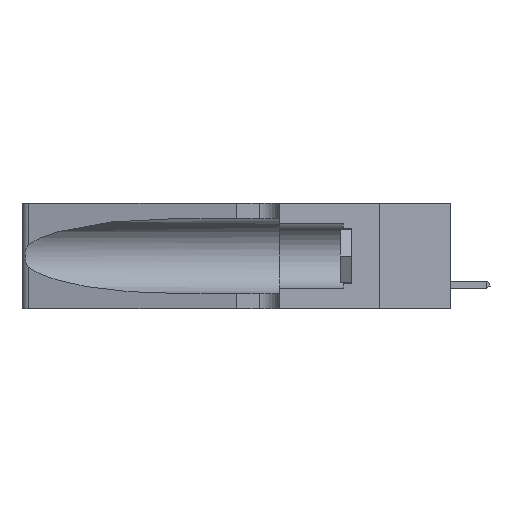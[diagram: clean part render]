
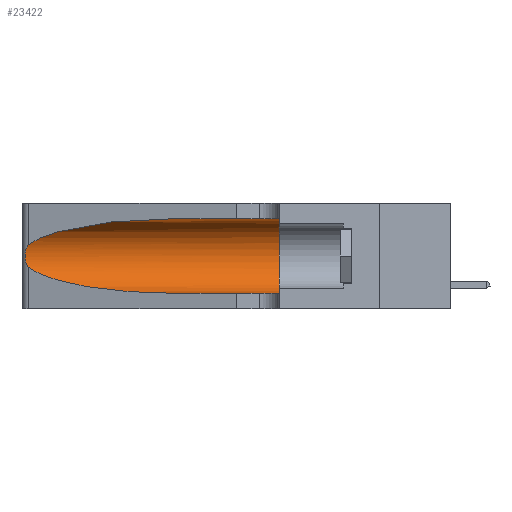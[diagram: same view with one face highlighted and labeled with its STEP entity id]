
A CAD part, left-side view. The second image highlights one B-rep face of the part: STEP entity #23422.
In plain terms, the highlighted cylindrical face has radius 3.308 mm (diameter 6.617 mm), a partial arc.
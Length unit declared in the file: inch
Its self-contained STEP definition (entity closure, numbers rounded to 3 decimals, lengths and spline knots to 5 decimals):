
#746 = ORIENTED_EDGE ( 'NONE', *, *, #5344, .F. ) ;
#1196 = CARTESIAN_POINT ( 'NONE',  ( 0.1305, 1.61858, 0.31525 ) ) ;
#1233 = VECTOR ( 'NONE', #22674, 39.37008 ) ;
#1549 = CARTESIAN_POINT ( 'NONE',  ( 0.25787, 1.23484, 0.2124 ) ) ;
#1666 = CARTESIAN_POINT ( 'NONE',  ( 0.25639, 1.23184, 0.21858 ) ) ;
#1991 = CARTESIAN_POINT ( 'NONE',  ( 0.1305, 0.72297, 0.05475 ) ) ;
#2087 = ORIENTED_EDGE ( 'NONE', *, *, #8302, .F. ) ;
#3786 = CARTESIAN_POINT ( 'NONE',  ( 0.18966, 0.96281, 0.31525 ) ) ;
#3876 = VERTEX_POINT ( 'NONE', #1991 ) ;
#3996 = VECTOR ( 'NONE', #4857, 39.37008 ) ;
#4454 = DIRECTION ( 'NONE',  ( 0., -1., 0. ) ) ;
#4857 = DIRECTION ( 'NONE',  ( 0., -1., 0. ) ) ;
#5344 = EDGE_CURVE ( 'NONE', #15802, #11603, #7976, .T. ) ;
#5470 = ORIENTED_EDGE ( 'NONE', *, *, #15708, .T. ) ;
#5559 = CARTESIAN_POINT ( 'NONE',  ( 0.25487, 1.22718, 0.22369 ) ) ;
#5665 = CARTESIAN_POINT ( 'NONE',  ( 0.25555, 1.22994, 0.2215 ) ) ;
#5696 = FACE_OUTER_BOUND ( 'NONE', #6865, .T. ) ;
#6238 = CARTESIAN_POINT ( 'NONE',  ( 0.25487, 1.22718, 0.22369 ) ) ;
#6282 = CARTESIAN_POINT ( 'NONE',  ( 0.25639, 1.23186, 0.15144 ) ) ;
#6865 = EDGE_LOOP ( 'NONE', ( #13003, #8755, #25587, #5470, #746, #2087 ) ) ;
#7184 = VERTEX_POINT ( 'NONE', #26812 ) ;
#7434 = CARTESIAN_POINT ( 'NONE',  ( 0.1305, 0.72297, 0.05475 ) ) ;
#7505 = CARTESIAN_POINT ( 'NONE',  ( 0.1305, 0.35, 0.185 ) ) ;
#7605 = DIRECTION ( 'NONE',  ( 0., 0., 1. ) ) ;
#7976 = CIRCLE ( 'NONE', #21541, 0.13025 ) ;
#8302 = EDGE_CURVE ( 'NONE', #19024, #15802, #31483, .T. ) ;
#8755 = ORIENTED_EDGE ( 'NONE', *, *, #11202, .T. ) ;
#8813 = CARTESIAN_POINT ( 'NONE',  ( 0.25487, 1.22718, 0.14631 ) ) ;
#9220 = CARTESIAN_POINT ( 'NONE',  ( 0.2373, 1.15595, 0.28018 ) ) ;
#9423 = CARTESIAN_POINT ( 'NONE',  ( 0.1305, 1.61858, 0.185 ) ) ;
#9803 =( BOUNDED_CURVE ( )  B_SPLINE_CURVE ( 3, ( #24480, #3786, #9220, #6238 ),
 .UNSPECIFIED., .F., .F. ) 
 B_SPLINE_CURVE_WITH_KNOTS ( ( 4, 4 ),
 ( 1.5708, 2.84003 ),
 .UNSPECIFIED. ) 
 CURVE ( )  GEOMETRIC_REPRESENTATION_ITEM ( )  RATIONAL_B_SPLINE_CURVE ( ( 1., 0.87, 0.87, 1. ) ) 
 REPRESENTATION_ITEM ( '' )  );
#11202 = EDGE_CURVE ( 'NONE', #28023, #7184, #19476, .T. ) ;
#11603 = VERTEX_POINT ( 'NONE', #31633 ) ;
#11711 = CARTESIAN_POINT ( 'NONE',  ( 0.26075, 1.23896, 0.19203 ) ) ;
#12378 = CARTESIAN_POINT ( 'NONE',  ( 0.1305, 1.61858, 0.05475 ) ) ;
#12766 = CARTESIAN_POINT ( 'NONE',  ( 0.25487, 1.22718, 0.22369 ) ) ;
#13003 = ORIENTED_EDGE ( 'NONE', *, *, #30274, .T. ) ;
#13230 = CYLINDRICAL_SURFACE ( 'NONE', #30563, 0.13025 ) ;
#15162 = CARTESIAN_POINT ( 'NONE',  ( 0.1305, 0.35, 0.31525 ) ) ;
#15708 = EDGE_CURVE ( 'NONE', #3876, #11603, #16445, .T. ) ;
#15802 = VERTEX_POINT ( 'NONE', #15162 ) ;
#16445 = LINE ( 'NONE', #12378, #1233 ) ;
#19024 = VERTEX_POINT ( 'NONE', #32672 ) ;
#19476 = B_SPLINE_CURVE_WITH_KNOTS ( 'NONE', 3,
 ( #5559, #5665, #1666, #1549, #32086, #26887, #11711, #29715, #22019, #29482, #24412, #6282, #24525, #8813 ),
 .UNSPECIFIED., .F., .F.,
 ( 4, 2, 2, 2, 2, 2, 4 ),
 ( 0., 0.00027, 0.00053, 0.00107, 0.0016, 0.00187, 0.00214 ),
 .UNSPECIFIED. ) ;
#19629 = CARTESIAN_POINT ( 'NONE',  ( 0.25487, 1.22718, 0.14631 ) ) ;
#21541 = AXIS2_PLACEMENT_3D ( 'NONE', #7505, #25317, #7605 ) ;
#22019 = CARTESIAN_POINT ( 'NONE',  ( 0.26017, 1.23833, 0.17102 ) ) ;
#22316 = CARTESIAN_POINT ( 'NONE',  ( 0.18966, 0.96281, 0.05475 ) ) ;
#22674 = DIRECTION ( 'NONE',  ( 0., -1., 0. ) ) ;
#23422 = ADVANCED_FACE ( 'NONE', ( #5696 ), #13230, .F. ) ;
#24164 = EDGE_CURVE ( 'NONE', #7184, #3876, #25910, .T. ) ;
#24412 = CARTESIAN_POINT ( 'NONE',  ( 0.25789, 1.23486, 0.15765 ) ) ;
#24480 = CARTESIAN_POINT ( 'NONE',  ( 0.1305, 0.72297, 0.31525 ) ) ;
#24525 = CARTESIAN_POINT ( 'NONE',  ( 0.25555, 1.22993, 0.14849 ) ) ;
#25317 = DIRECTION ( 'NONE',  ( 0., 1., 0. ) ) ;
#25587 = ORIENTED_EDGE ( 'NONE', *, *, #24164, .T. ) ;
#25910 =( BOUNDED_CURVE ( )  B_SPLINE_CURVE ( 3, ( #19629, #32511, #22316, #7434 ),
 .UNSPECIFIED., .F., .F. ) 
 B_SPLINE_CURVE_WITH_KNOTS ( ( 4, 4 ),
 ( 3.44316, 4.71239 ),
 .UNSPECIFIED. ) 
 CURVE ( )  GEOMETRIC_REPRESENTATION_ITEM ( )  RATIONAL_B_SPLINE_CURVE ( ( 1., 0.87, 0.87, 1. ) ) 
 REPRESENTATION_ITEM ( '' )  );
#26812 = CARTESIAN_POINT ( 'NONE',  ( 0.25487, 1.22718, 0.14631 ) ) ;
#26887 = CARTESIAN_POINT ( 'NONE',  ( 0.26018, 1.23835, 0.19895 ) ) ;
#27485 = DIRECTION ( 'NONE',  ( 0., 0., -1. ) ) ;
#28023 = VERTEX_POINT ( 'NONE', #12766 ) ;
#29482 = CARTESIAN_POINT ( 'NONE',  ( 0.25856, 1.23593, 0.16098 ) ) ;
#29715 = CARTESIAN_POINT ( 'NONE',  ( 0.26075, 1.23896, 0.178 ) ) ;
#30274 = EDGE_CURVE ( 'NONE', #19024, #28023, #9803, .T. ) ;
#30563 = AXIS2_PLACEMENT_3D ( 'NONE', #9423, #4454, #27485 ) ;
#31483 = LINE ( 'NONE', #1196, #3996 ) ;
#31633 = CARTESIAN_POINT ( 'NONE',  ( 0.1305, 0.35, 0.05475 ) ) ;
#32086 = CARTESIAN_POINT ( 'NONE',  ( 0.25854, 1.2359, 0.20912 ) ) ;
#32511 = CARTESIAN_POINT ( 'NONE',  ( 0.2373, 1.15595, 0.08982 ) ) ;
#32672 = CARTESIAN_POINT ( 'NONE',  ( 0.1305, 0.72297, 0.31525 ) ) ;
